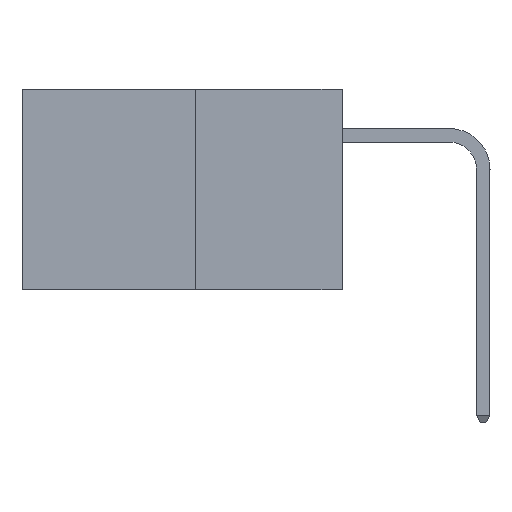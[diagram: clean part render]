
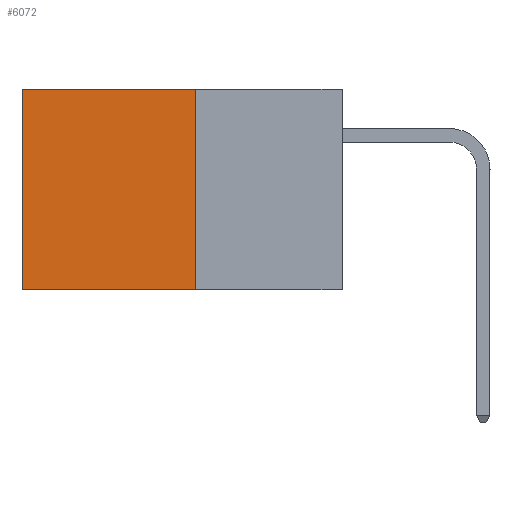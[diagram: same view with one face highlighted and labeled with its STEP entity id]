
A CAD part, left-side view. The second image highlights one B-rep face of the part: STEP entity #6072.
In plain terms, the highlighted planar face has unit normal (-1, 0, 0).
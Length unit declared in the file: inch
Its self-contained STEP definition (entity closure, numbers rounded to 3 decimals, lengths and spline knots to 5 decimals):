
#248 = DIRECTION ( 'NONE',  ( 0., 1., 0. ) ) ;
#316 = ORIENTED_EDGE ( 'NONE', *, *, #5095, .F. ) ;
#721 = VECTOR ( 'NONE', #10731, 39.37008 ) ;
#1350 = VECTOR ( 'NONE', #10267, 39.37008 ) ;
#1480 = EDGE_CURVE ( 'NONE', #8870, #3840, #13649, .T. ) ;
#2036 = FACE_OUTER_BOUND ( 'NONE', #13703, .T. ) ;
#2828 = LINE ( 'NONE', #2915, #6124 ) ;
#2915 = CARTESIAN_POINT ( 'NONE',  ( 0.277, 0.27, -0.37 ) ) ;
#3067 = CARTESIAN_POINT ( 'NONE',  ( 0.277, 0.27, -0.37 ) ) ;
#3783 = VERTEX_POINT ( 'NONE', #14326 ) ;
#3840 = VERTEX_POINT ( 'NONE', #10588 ) ;
#4745 = DIRECTION ( 'NONE',  ( 0., 0., -1. ) ) ;
#5095 = EDGE_CURVE ( 'NONE', #8979, #3840, #2828, .T. ) ;
#5473 = EDGE_CURVE ( 'NONE', #3783, #8870, #10897, .T. ) ;
#5903 = DIRECTION ( 'NONE',  ( 1., 0., 0. ) ) ;
#6072 = ADVANCED_FACE ( 'NONE', ( #2036 ), #8960, .F. ) ;
#6124 = VECTOR ( 'NONE', #248, 39.37008 ) ;
#6252 = AXIS2_PLACEMENT_3D ( 'NONE', #3067, #5903, #4745 ) ;
#6709 = CARTESIAN_POINT ( 'NONE',  ( 0.277, 0.27, -0.37 ) ) ;
#6751 = ORIENTED_EDGE ( 'NONE', *, *, #5473, .T. ) ;
#7566 = EDGE_CURVE ( 'NONE', #3783, #8979, #10274, .T. ) ;
#7619 = VECTOR ( 'NONE', #14644, 39.37008 ) ;
#8594 = CARTESIAN_POINT ( 'NONE',  ( 0.277, 0.59, 0. ) ) ;
#8849 = CARTESIAN_POINT ( 'NONE',  ( 0.277, 0.27, -0.37 ) ) ;
#8870 = VERTEX_POINT ( 'NONE', #8594 ) ;
#8960 = PLANE ( 'NONE',  #6252 ) ;
#8979 = VERTEX_POINT ( 'NONE', #8849 ) ;
#10267 = DIRECTION ( 'NONE',  ( 0., 1., 0. ) ) ;
#10274 = LINE ( 'NONE', #6709, #721 ) ;
#10339 = CARTESIAN_POINT ( 'NONE',  ( 0.277, 0.27, 0. ) ) ;
#10588 = CARTESIAN_POINT ( 'NONE',  ( 0.277, 0.59, -0.37 ) ) ;
#10731 = DIRECTION ( 'NONE',  ( 0., 0., -1. ) ) ;
#10897 = LINE ( 'NONE', #10339, #1350 ) ;
#10968 = ORIENTED_EDGE ( 'NONE', *, *, #1480, .T. ) ;
#13649 = LINE ( 'NONE', #14940, #7619 ) ;
#13703 = EDGE_LOOP ( 'NONE', ( #10968, #316, #14905, #6751 ) ) ;
#14326 = CARTESIAN_POINT ( 'NONE',  ( 0.277, 0.27, 0. ) ) ;
#14644 = DIRECTION ( 'NONE',  ( 0., 0., -1. ) ) ;
#14905 = ORIENTED_EDGE ( 'NONE', *, *, #7566, .F. ) ;
#14940 = CARTESIAN_POINT ( 'NONE',  ( 0.277, 0.59, -0.37 ) ) ;
